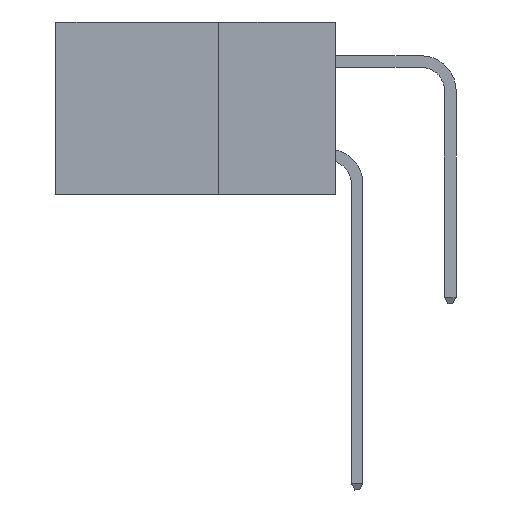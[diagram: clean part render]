
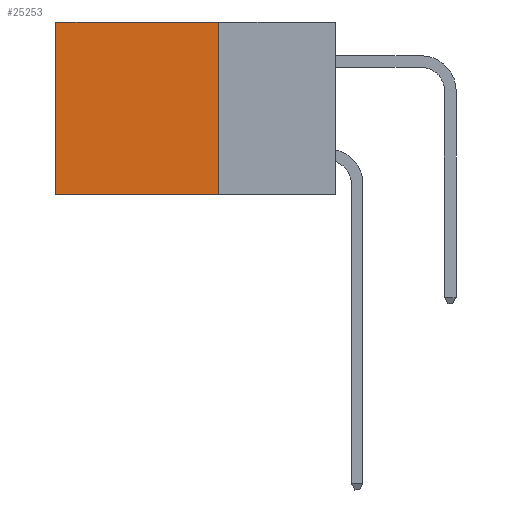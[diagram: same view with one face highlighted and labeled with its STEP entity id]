
A CAD part, left-side view. The second image highlights one B-rep face of the part: STEP entity #25253.
In plain terms, the highlighted planar face has unit normal (-1, 0, 0).
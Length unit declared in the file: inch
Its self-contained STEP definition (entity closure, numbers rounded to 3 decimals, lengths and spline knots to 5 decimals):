
#1402 = CARTESIAN_POINT ( 'NONE',  ( 0.2875, 0.25, 0. ) ) ;
#2773 = CARTESIAN_POINT ( 'NONE',  ( 0.2875, 0.6, -0.37 ) ) ;
#3939 = EDGE_LOOP ( 'NONE', ( #30376, #27632, #25651, #13517 ) ) ;
#5908 = LINE ( 'NONE', #26607, #28862 ) ;
#6433 = VERTEX_POINT ( 'NONE', #7278 ) ;
#6866 = DIRECTION ( 'NONE',  ( 1., 0., 0. ) ) ;
#7278 = CARTESIAN_POINT ( 'NONE',  ( 0.2875, 0.6, 0. ) ) ;
#9080 = DIRECTION ( 'NONE',  ( 0., 1., 0. ) ) ;
#9854 = EDGE_CURVE ( 'NONE', #6433, #23830, #5908, .T. ) ;
#12699 = EDGE_CURVE ( 'NONE', #24069, #19718, #15352, .T. ) ;
#13517 = ORIENTED_EDGE ( 'NONE', *, *, #22123, .T. ) ;
#13596 = CARTESIAN_POINT ( 'NONE',  ( 0.2875, 0.25, -0.37 ) ) ;
#14216 = PLANE ( 'NONE',  #32700 ) ;
#15352 = LINE ( 'NONE', #18087, #33253 ) ;
#16484 = VECTOR ( 'NONE', #19817, 39.37008 ) ;
#17284 = CARTESIAN_POINT ( 'NONE',  ( 0.2875, 0.25, 0. ) ) ;
#18087 = CARTESIAN_POINT ( 'NONE',  ( 0.2875, 0.25, 0. ) ) ;
#19151 = CARTESIAN_POINT ( 'NONE',  ( 0.2875, 0.25, -0.37 ) ) ;
#19325 = LINE ( 'NONE', #19151, #16484 ) ;
#19718 = VERTEX_POINT ( 'NONE', #13596 ) ;
#19817 = DIRECTION ( 'NONE',  ( 0., 1., 0. ) ) ;
#20633 = DIRECTION ( 'NONE',  ( 0., 0., -1. ) ) ;
#22077 = LINE ( 'NONE', #32496, #27733 ) ;
#22123 = EDGE_CURVE ( 'NONE', #24069, #6433, #22077, .T. ) ;
#23830 = VERTEX_POINT ( 'NONE', #2773 ) ;
#24069 = VERTEX_POINT ( 'NONE', #1402 ) ;
#25253 = ADVANCED_FACE ( 'NONE', ( #32672 ), #14216, .F. ) ;
#25651 = ORIENTED_EDGE ( 'NONE', *, *, #12699, .F. ) ;
#26451 = DIRECTION ( 'NONE',  ( 0., 0., -1. ) ) ;
#26607 = CARTESIAN_POINT ( 'NONE',  ( 0.2875, 0.6, 0. ) ) ;
#27396 = DIRECTION ( 'NONE',  ( 0., 0., -1. ) ) ;
#27632 = ORIENTED_EDGE ( 'NONE', *, *, #28341, .F. ) ;
#27733 = VECTOR ( 'NONE', #9080, 39.37008 ) ;
#28341 = EDGE_CURVE ( 'NONE', #19718, #23830, #19325, .T. ) ;
#28862 = VECTOR ( 'NONE', #26451, 39.37008 ) ;
#30376 = ORIENTED_EDGE ( 'NONE', *, *, #9854, .T. ) ;
#32496 = CARTESIAN_POINT ( 'NONE',  ( 0.2875, 0.25, 0. ) ) ;
#32672 = FACE_OUTER_BOUND ( 'NONE', #3939, .T. ) ;
#32700 = AXIS2_PLACEMENT_3D ( 'NONE', #17284, #6866, #27396 ) ;
#33253 = VECTOR ( 'NONE', #20633, 39.37008 ) ;
